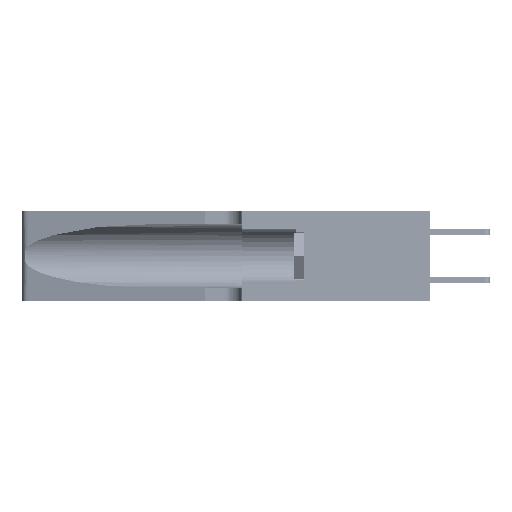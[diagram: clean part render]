
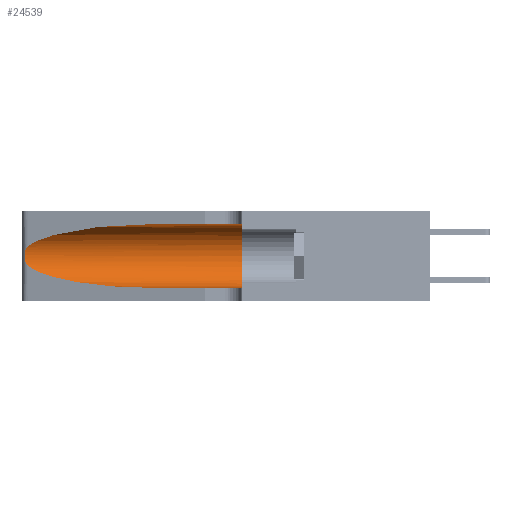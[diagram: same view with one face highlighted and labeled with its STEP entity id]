
A CAD part, left-side view. The second image highlights one B-rep face of the part: STEP entity #24539.
In plain terms, the highlighted cylindrical face has radius 3.308 mm (diameter 6.617 mm), a partial arc.
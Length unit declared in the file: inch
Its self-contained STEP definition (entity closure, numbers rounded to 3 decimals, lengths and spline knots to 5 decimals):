
#685 = CARTESIAN_POINT ( 'NONE',  ( 0.1305, 0.72297, 0.31525 ) ) ;
#1034 = VERTEX_POINT ( 'NONE', #35264 ) ;
#1325 = CARTESIAN_POINT ( 'NONE',  ( 0.25487, 1.22718, 0.22369 ) ) ;
#1748 = EDGE_LOOP ( 'NONE', ( #40333, #11816, #15640, #11291, #25154, #2761 ) ) ;
#1806 = EDGE_CURVE ( 'NONE', #37711, #8370, #18530, .T. ) ;
#2551 = CIRCLE ( 'NONE', #33050, 0.13025 ) ;
#2695 = CARTESIAN_POINT ( 'NONE',  ( 0.26018, 1.23835, 0.19895 ) ) ;
#2761 = ORIENTED_EDGE ( 'NONE', *, *, #17952, .F. ) ;
#4075 = CARTESIAN_POINT ( 'NONE',  ( 0.18966, 0.96281, 0.31525 ) ) ;
#4231 = CARTESIAN_POINT ( 'NONE',  ( 0.1305, 0.72297, 0.31525 ) ) ;
#5081 = DIRECTION ( 'NONE',  ( 0., -1., 0. ) ) ;
#6039 = EDGE_CURVE ( 'NONE', #8370, #1034, #41553, .T. ) ;
#6124 = CARTESIAN_POINT ( 'NONE',  ( 0.26075, 1.23896, 0.178 ) ) ;
#6221 = CARTESIAN_POINT ( 'NONE',  ( 0.1305, 1.61858, 0.31525 ) ) ;
#7812 = CARTESIAN_POINT ( 'NONE',  ( 0.25487, 1.22718, 0.14631 ) ) ;
#8370 = VERTEX_POINT ( 'NONE', #18418 ) ;
#8843 = CARTESIAN_POINT ( 'NONE',  ( 0.1305, 0.35, 0.185 ) ) ;
#9258 = VERTEX_POINT ( 'NONE', #19428 ) ;
#9485 = CARTESIAN_POINT ( 'NONE',  ( 0.25787, 1.23484, 0.2124 ) ) ;
#9787 = LINE ( 'NONE', #6221, #32438 ) ;
#10130 = EDGE_CURVE ( 'NONE', #9258, #31284, #29310, .T. ) ;
#11291 = ORIENTED_EDGE ( 'NONE', *, *, #10130, .T. ) ;
#11535 = DIRECTION ( 'NONE',  ( 0., 0., -1. ) ) ;
#11752 = CARTESIAN_POINT ( 'NONE',  ( 0.25555, 1.22994, 0.2215 ) ) ;
#11816 = ORIENTED_EDGE ( 'NONE', *, *, #6039, .T. ) ;
#12064 = DIRECTION ( 'NONE',  ( 0., 0., 1. ) ) ;
#12963 = CARTESIAN_POINT ( 'NONE',  ( 0.25789, 1.23486, 0.15765 ) ) ;
#13214 = VERTEX_POINT ( 'NONE', #39233 ) ;
#13938 = CARTESIAN_POINT ( 'NONE',  ( 0.2373, 1.15595, 0.28018 ) ) ;
#13992 = CARTESIAN_POINT ( 'NONE',  ( 0.18966, 0.96281, 0.05475 ) ) ;
#15279 = CARTESIAN_POINT ( 'NONE',  ( 0.26017, 1.23833, 0.17102 ) ) ;
#15406 = CARTESIAN_POINT ( 'NONE',  ( 0.26075, 1.23896, 0.19203 ) ) ;
#15640 = ORIENTED_EDGE ( 'NONE', *, *, #41241, .T. ) ;
#15900 = DIRECTION ( 'NONE',  ( 0., -1., 0. ) ) ;
#16213 = VECTOR ( 'NONE', #32837, 39.37008 ) ;
#17058 = CARTESIAN_POINT ( 'NONE',  ( 0.2373, 1.15595, 0.08982 ) ) ;
#17952 = EDGE_CURVE ( 'NONE', #37711, #13214, #9787, .T. ) ;
#18418 = CARTESIAN_POINT ( 'NONE',  ( 0.25487, 1.22718, 0.22369 ) ) ;
#18530 =( BOUNDED_CURVE ( )  B_SPLINE_CURVE ( 3, ( #4231, #4075, #13938, #26749 ),
 .UNSPECIFIED., .F., .F. ) 
 B_SPLINE_CURVE_WITH_KNOTS ( ( 4, 4 ),
 ( 1.5708, 2.84003 ),
 .UNSPECIFIED. ) 
 CURVE ( )  GEOMETRIC_REPRESENTATION_ITEM ( )  RATIONAL_B_SPLINE_CURVE ( ( 1., 0.87, 0.87, 1. ) ) 
 REPRESENTATION_ITEM ( '' )  );
#19428 = CARTESIAN_POINT ( 'NONE',  ( 0.1305, 0.72297, 0.05475 ) ) ;
#19584 = CYLINDRICAL_SURFACE ( 'NONE', #37473, 0.13025 ) ;
#20726 = CARTESIAN_POINT ( 'NONE',  ( 0.1305, 1.61858, 0.185 ) ) ;
#22033 = CARTESIAN_POINT ( 'NONE',  ( 0.25854, 1.2359, 0.20912 ) ) ;
#22167 = CARTESIAN_POINT ( 'NONE',  ( 0.25639, 1.23184, 0.21858 ) ) ;
#22548 = EDGE_CURVE ( 'NONE', #13214, #31284, #2551, .T. ) ;
#24539 = ADVANCED_FACE ( 'NONE', ( #30166 ), #19584, .F. ) ;
#24625 = DIRECTION ( 'NONE',  ( 0., 1., 0. ) ) ;
#24782 =( BOUNDED_CURVE ( )  B_SPLINE_CURVE ( 3, ( #7812, #17058, #13992, #40054 ),
 .UNSPECIFIED., .F., .T. ) 
 B_SPLINE_CURVE_WITH_KNOTS ( ( 4, 4 ),
 ( 3.44316, 4.71239 ),
 .UNSPECIFIED. ) 
 CURVE ( )  GEOMETRIC_REPRESENTATION_ITEM ( )  RATIONAL_B_SPLINE_CURVE ( ( 1., 0.87, 0.87, 1. ) ) 
 REPRESENTATION_ITEM ( '' )  );
#25154 = ORIENTED_EDGE ( 'NONE', *, *, #22548, .F. ) ;
#26749 = CARTESIAN_POINT ( 'NONE',  ( 0.25487, 1.22718, 0.22369 ) ) ;
#29164 = CARTESIAN_POINT ( 'NONE',  ( 0.25639, 1.23186, 0.15144 ) ) ;
#29310 = LINE ( 'NONE', #29865, #16213 ) ;
#29431 = CARTESIAN_POINT ( 'NONE',  ( 0.25555, 1.22993, 0.14849 ) ) ;
#29865 = CARTESIAN_POINT ( 'NONE',  ( 0.1305, 1.61858, 0.05475 ) ) ;
#30166 = FACE_OUTER_BOUND ( 'NONE', #1748, .T. ) ;
#31284 = VERTEX_POINT ( 'NONE', #35544 ) ;
#32438 = VECTOR ( 'NONE', #15900, 39.37008 ) ;
#32837 = DIRECTION ( 'NONE',  ( 0., -1., 0. ) ) ;
#33050 = AXIS2_PLACEMENT_3D ( 'NONE', #8843, #24625, #12064 ) ;
#35243 = CARTESIAN_POINT ( 'NONE',  ( 0.25487, 1.22718, 0.14631 ) ) ;
#35264 = CARTESIAN_POINT ( 'NONE',  ( 0.25487, 1.22718, 0.14631 ) ) ;
#35544 = CARTESIAN_POINT ( 'NONE',  ( 0.1305, 0.35, 0.05475 ) ) ;
#35770 = CARTESIAN_POINT ( 'NONE',  ( 0.25856, 1.23593, 0.16098 ) ) ;
#37473 = AXIS2_PLACEMENT_3D ( 'NONE', #20726, #5081, #11535 ) ;
#37711 = VERTEX_POINT ( 'NONE', #685 ) ;
#39233 = CARTESIAN_POINT ( 'NONE',  ( 0.1305, 0.35, 0.31525 ) ) ;
#40054 = CARTESIAN_POINT ( 'NONE',  ( 0.1305, 0.72297, 0.05475 ) ) ;
#40333 = ORIENTED_EDGE ( 'NONE', *, *, #1806, .T. ) ;
#41241 = EDGE_CURVE ( 'NONE', #1034, #9258, #24782, .T. ) ;
#41553 = B_SPLINE_CURVE_WITH_KNOTS ( 'NONE', 3,
 ( #1325, #11752, #22167, #9485, #22033, #2695, #15406, #6124, #15279, #35770, #12963, #29164, #29431, #35243 ),
 .UNSPECIFIED., .F., .F.,
 ( 4, 2, 2, 2, 2, 2, 4 ),
 ( 0., 0.00027, 0.00053, 0.00107, 0.0016, 0.00187, 0.00214 ),
 .UNSPECIFIED. ) ;
